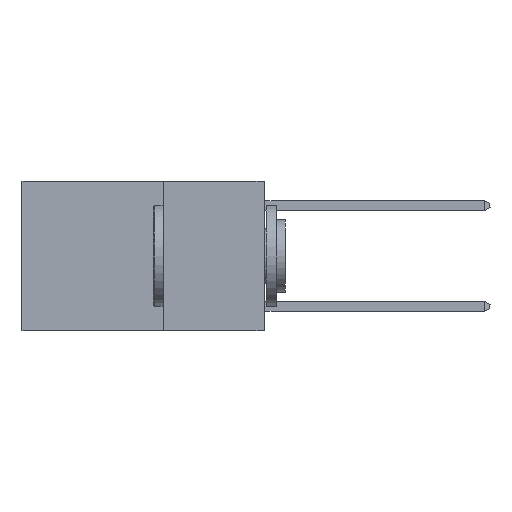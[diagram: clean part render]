
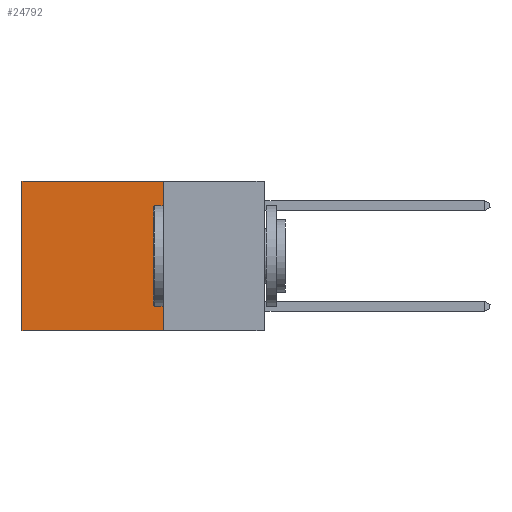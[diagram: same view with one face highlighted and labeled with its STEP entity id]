
A CAD part, left-side view. The second image highlights one B-rep face of the part: STEP entity #24792.
In plain terms, the highlighted planar face has unit normal (-1, 0, 0).
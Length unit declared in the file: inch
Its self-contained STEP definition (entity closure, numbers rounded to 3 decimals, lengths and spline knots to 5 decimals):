
#638 = CARTESIAN_POINT ( 'NONE',  ( 0.2625, 0.25, 0. ) ) ;
#781 = DIRECTION ( 'NONE',  ( 1., 0., 0. ) ) ;
#2060 = EDGE_CURVE ( 'NONE', #26600, #6586, #17590, .T. ) ;
#2958 = DIRECTION ( 'NONE',  ( 0., 1., 0. ) ) ;
#2994 = VECTOR ( 'NONE', #24876, 39.37008 ) ;
#3472 = VECTOR ( 'NONE', #2958, 39.37008 ) ;
#4762 = AXIS2_PLACEMENT_3D ( 'NONE', #638, #781, #4801 ) ;
#4801 = DIRECTION ( 'NONE',  ( 0., 0., -1. ) ) ;
#6518 = CARTESIAN_POINT ( 'NONE',  ( 0.2625, 0.6, -0.37 ) ) ;
#6586 = VERTEX_POINT ( 'NONE', #6518 ) ;
#8442 = ORIENTED_EDGE ( 'NONE', *, *, #2060, .F. ) ;
#9318 = EDGE_LOOP ( 'NONE', ( #26461, #8442, #19129, #20292 ) ) ;
#9902 = EDGE_CURVE ( 'NONE', #11688, #6586, #18609, .T. ) ;
#11688 = VERTEX_POINT ( 'NONE', #17220 ) ;
#11693 = CARTESIAN_POINT ( 'NONE',  ( 0.2625, 0.6, 0. ) ) ;
#11719 = VECTOR ( 'NONE', #25090, 39.37008 ) ;
#11783 = LINE ( 'NONE', #27122, #11719 ) ;
#12473 = VECTOR ( 'NONE', #14009, 39.37008 ) ;
#13480 = FACE_OUTER_BOUND ( 'NONE', #9318, .T. ) ;
#13520 = VERTEX_POINT ( 'NONE', #21684 ) ;
#14009 = DIRECTION ( 'NONE',  ( 0., 0., -1. ) ) ;
#16079 = EDGE_CURVE ( 'NONE', #13520, #26600, #11783, .T. ) ;
#16508 = EDGE_CURVE ( 'NONE', #13520, #11688, #25016, .T. ) ;
#17220 = CARTESIAN_POINT ( 'NONE',  ( 0.2625, 0.6, 0. ) ) ;
#17399 = CARTESIAN_POINT ( 'NONE',  ( 0.2625, 0.25, -0.37 ) ) ;
#17590 = LINE ( 'NONE', #22736, #3472 ) ;
#18609 = LINE ( 'NONE', #11693, #12473 ) ;
#19129 = ORIENTED_EDGE ( 'NONE', *, *, #16079, .F. ) ;
#20274 = PLANE ( 'NONE',  #4762 ) ;
#20292 = ORIENTED_EDGE ( 'NONE', *, *, #16508, .T. ) ;
#21684 = CARTESIAN_POINT ( 'NONE',  ( 0.2625, 0.25, 0. ) ) ;
#22736 = CARTESIAN_POINT ( 'NONE',  ( 0.2625, 0.25, -0.37 ) ) ;
#22984 = CARTESIAN_POINT ( 'NONE',  ( 0.2625, 0.25, 0. ) ) ;
#24792 = ADVANCED_FACE ( 'NONE', ( #13480 ), #20274, .F. ) ;
#24876 = DIRECTION ( 'NONE',  ( 0., 1., 0. ) ) ;
#25016 = LINE ( 'NONE', #22984, #2994 ) ;
#25090 = DIRECTION ( 'NONE',  ( 0., 0., -1. ) ) ;
#26461 = ORIENTED_EDGE ( 'NONE', *, *, #9902, .T. ) ;
#26600 = VERTEX_POINT ( 'NONE', #17399 ) ;
#27122 = CARTESIAN_POINT ( 'NONE',  ( 0.2625, 0.25, 0. ) ) ;
